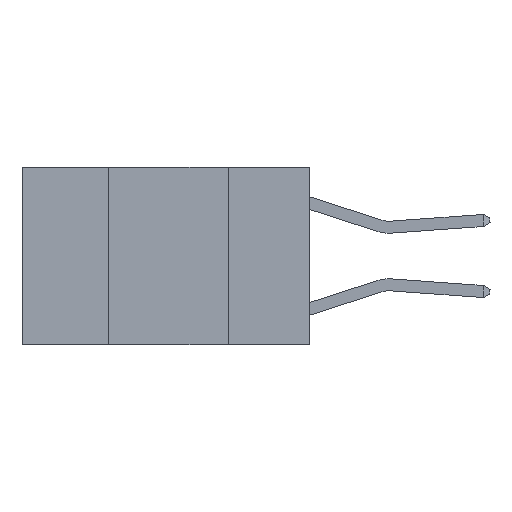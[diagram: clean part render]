
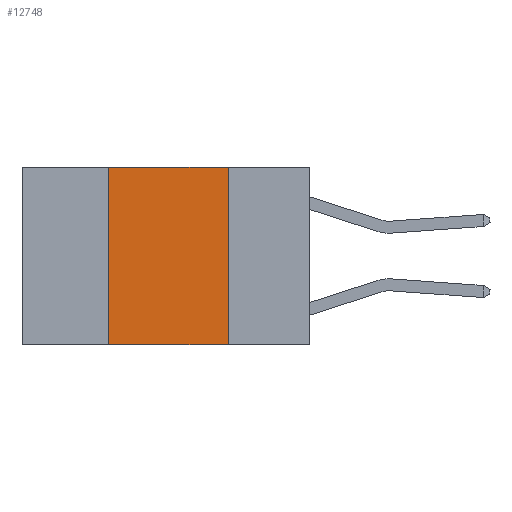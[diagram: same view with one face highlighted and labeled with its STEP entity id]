
A CAD part, left-side view. The second image highlights one B-rep face of the part: STEP entity #12748.
In plain terms, the highlighted planar face has unit normal (-1, 0, 0).
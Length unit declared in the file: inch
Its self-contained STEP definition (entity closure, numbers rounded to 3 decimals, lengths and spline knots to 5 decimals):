
#98 = EDGE_LOOP ( 'NONE', ( #7782, #16408, #4119, #13326 ) ) ;
#409 = VERTEX_POINT ( 'NONE', #4088 ) ;
#938 = EDGE_CURVE ( 'NONE', #409, #2877, #5175, .T. ) ;
#2574 = VECTOR ( 'NONE', #13694, 39.37008 ) ;
#2650 = DIRECTION ( 'NONE',  ( 0., 0., -1. ) ) ;
#2838 = CARTESIAN_POINT ( 'NONE',  ( 0., 0.17, -0.37 ) ) ;
#2877 = VERTEX_POINT ( 'NONE', #2838 ) ;
#3086 = FACE_OUTER_BOUND ( 'NONE', #98, .T. ) ;
#3457 = EDGE_CURVE ( 'NONE', #409, #13774, #6023, .T. ) ;
#4088 = CARTESIAN_POINT ( 'NONE',  ( 0., 0.42, -0.37 ) ) ;
#4119 = ORIENTED_EDGE ( 'NONE', *, *, #3457, .F. ) ;
#4201 = VERTEX_POINT ( 'NONE', #15359 ) ;
#4555 = EDGE_CURVE ( 'NONE', #13774, #4201, #11378, .T. ) ;
#4718 = CARTESIAN_POINT ( 'NONE',  ( 0., 0.6, 0. ) ) ;
#4963 = DIRECTION ( 'NONE',  ( 0., -1., 0. ) ) ;
#5175 = LINE ( 'NONE', #10312, #10882 ) ;
#6023 = LINE ( 'NONE', #16219, #2574 ) ;
#7782 = ORIENTED_EDGE ( 'NONE', *, *, #10022, .F. ) ;
#8674 = CARTESIAN_POINT ( 'NONE',  ( 0., 0.42, 0. ) ) ;
#9339 = VECTOR ( 'NONE', #4963, 39.37008 ) ;
#10022 = EDGE_CURVE ( 'NONE', #4201, #2877, #11614, .T. ) ;
#10312 = CARTESIAN_POINT ( 'NONE',  ( 0., 0.6, -0.37 ) ) ;
#10610 = PLANE ( 'NONE',  #11576 ) ;
#10882 = VECTOR ( 'NONE', #15542, 39.37008 ) ;
#11378 = LINE ( 'NONE', #4718, #9339 ) ;
#11576 = AXIS2_PLACEMENT_3D ( 'NONE', #12047, #11797, #11884 ) ;
#11614 = LINE ( 'NONE', #13039, #13757 ) ;
#11797 = DIRECTION ( 'NONE',  ( 1., 0., 0. ) ) ;
#11884 = DIRECTION ( 'NONE',  ( 0., 0., -1. ) ) ;
#12047 = CARTESIAN_POINT ( 'NONE',  ( 0., 0.6, 0. ) ) ;
#12748 = ADVANCED_FACE ( 'NONE', ( #3086 ), #10610, .F. ) ;
#13039 = CARTESIAN_POINT ( 'NONE',  ( 0., 0.17, 0. ) ) ;
#13326 = ORIENTED_EDGE ( 'NONE', *, *, #938, .T. ) ;
#13694 = DIRECTION ( 'NONE',  ( 0., 0., 1. ) ) ;
#13757 = VECTOR ( 'NONE', #2650, 39.37008 ) ;
#13774 = VERTEX_POINT ( 'NONE', #8674 ) ;
#15359 = CARTESIAN_POINT ( 'NONE',  ( 0., 0.17, 0. ) ) ;
#15542 = DIRECTION ( 'NONE',  ( 0., -1., 0. ) ) ;
#16219 = CARTESIAN_POINT ( 'NONE',  ( 0., 0.42, 0. ) ) ;
#16408 = ORIENTED_EDGE ( 'NONE', *, *, #4555, .F. ) ;
